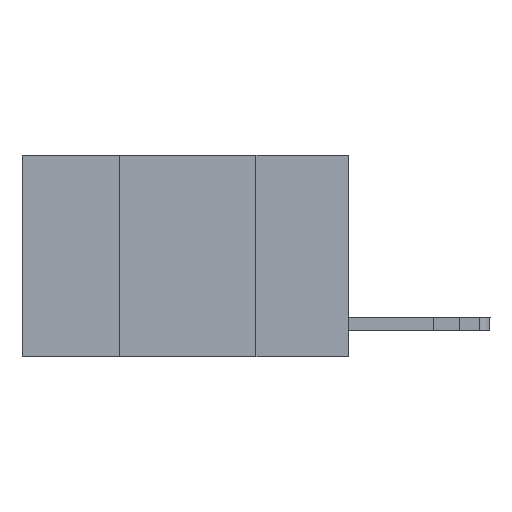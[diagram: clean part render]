
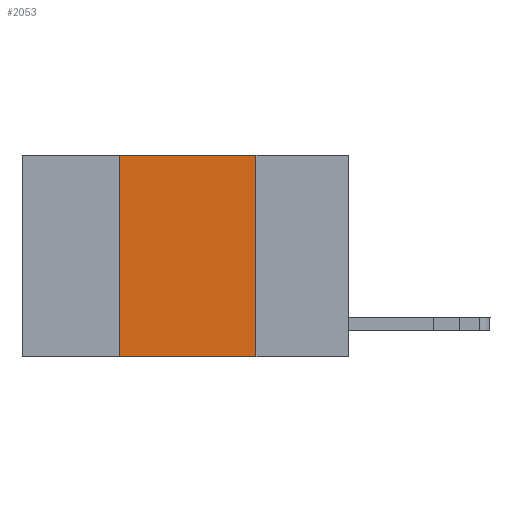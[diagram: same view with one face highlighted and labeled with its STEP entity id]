
A CAD part, left-side view. The second image highlights one B-rep face of the part: STEP entity #2053.
In plain terms, the highlighted planar face has unit normal (-1, 0, 0).
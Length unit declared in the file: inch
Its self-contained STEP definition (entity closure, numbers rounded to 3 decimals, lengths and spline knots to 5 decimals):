
#1277 = EDGE_LOOP ( 'NONE', ( #7251, #5032, #18038, #20586 ) ) ;
#1609 = DIRECTION ( 'NONE',  ( 0., 0., -1. ) ) ;
#1633 = VECTOR ( 'NONE', #14971, 39.37008 ) ;
#1765 = VERTEX_POINT ( 'NONE', #10247 ) ;
#1772 = LINE ( 'NONE', #16385, #10411 ) ;
#2053 = ADVANCED_FACE ( 'NONE', ( #15714 ), #10186, .F. ) ;
#3683 = EDGE_CURVE ( 'NONE', #16358, #20830, #5919, .T. ) ;
#4363 = DIRECTION ( 'NONE',  ( 0., -1., 0. ) ) ;
#4982 = VECTOR ( 'NONE', #1609, 39.37008 ) ;
#5032 = ORIENTED_EDGE ( 'NONE', *, *, #3683, .F. ) ;
#5246 = VERTEX_POINT ( 'NONE', #15027 ) ;
#5919 = LINE ( 'NONE', #16676, #9981 ) ;
#6220 = LINE ( 'NONE', #21789, #1633 ) ;
#6289 = CARTESIAN_POINT ( 'NONE',  ( 0., 0.6, 0. ) ) ;
#6516 = EDGE_CURVE ( 'NONE', #5246, #16358, #6220, .T. ) ;
#7251 = ORIENTED_EDGE ( 'NONE', *, *, #16164, .F. ) ;
#9807 = AXIS2_PLACEMENT_3D ( 'NONE', #6289, #14539, #18705 ) ;
#9981 = VECTOR ( 'NONE', #11996, 39.37008 ) ;
#10105 = LINE ( 'NONE', #15404, #4982 ) ;
#10186 = PLANE ( 'NONE',  #9807 ) ;
#10247 = CARTESIAN_POINT ( 'NONE',  ( 0., 0.17, -0.37 ) ) ;
#10411 = VECTOR ( 'NONE', #4363, 39.37008 ) ;
#10778 = CARTESIAN_POINT ( 'NONE',  ( 0., 0.42, 0. ) ) ;
#11996 = DIRECTION ( 'NONE',  ( 0., -1., 0. ) ) ;
#12935 = CARTESIAN_POINT ( 'NONE',  ( 0., 0.17, 0. ) ) ;
#14539 = DIRECTION ( 'NONE',  ( 1., 0., 0. ) ) ;
#14971 = DIRECTION ( 'NONE',  ( 0., 0., 1. ) ) ;
#15022 = EDGE_CURVE ( 'NONE', #5246, #1765, #1772, .T. ) ;
#15027 = CARTESIAN_POINT ( 'NONE',  ( 0., 0.42, -0.37 ) ) ;
#15404 = CARTESIAN_POINT ( 'NONE',  ( 0., 0.17, 0. ) ) ;
#15714 = FACE_OUTER_BOUND ( 'NONE', #1277, .T. ) ;
#16164 = EDGE_CURVE ( 'NONE', #20830, #1765, #10105, .T. ) ;
#16358 = VERTEX_POINT ( 'NONE', #10778 ) ;
#16385 = CARTESIAN_POINT ( 'NONE',  ( 0., 0.6, -0.37 ) ) ;
#16676 = CARTESIAN_POINT ( 'NONE',  ( 0., 0.6, 0. ) ) ;
#18038 = ORIENTED_EDGE ( 'NONE', *, *, #6516, .F. ) ;
#18705 = DIRECTION ( 'NONE',  ( 0., 0., -1. ) ) ;
#20586 = ORIENTED_EDGE ( 'NONE', *, *, #15022, .T. ) ;
#20830 = VERTEX_POINT ( 'NONE', #12935 ) ;
#21789 = CARTESIAN_POINT ( 'NONE',  ( 0., 0.42, 0. ) ) ;
